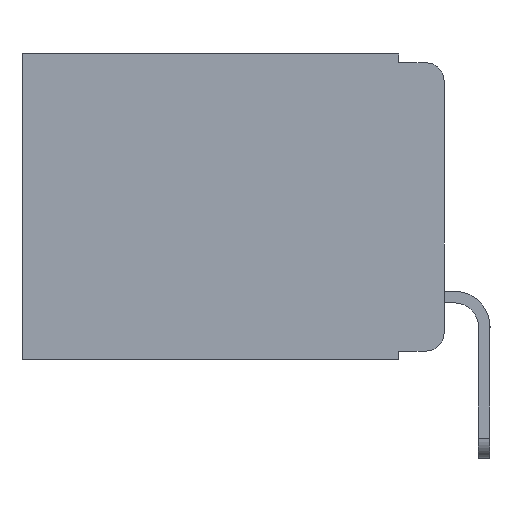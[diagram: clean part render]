
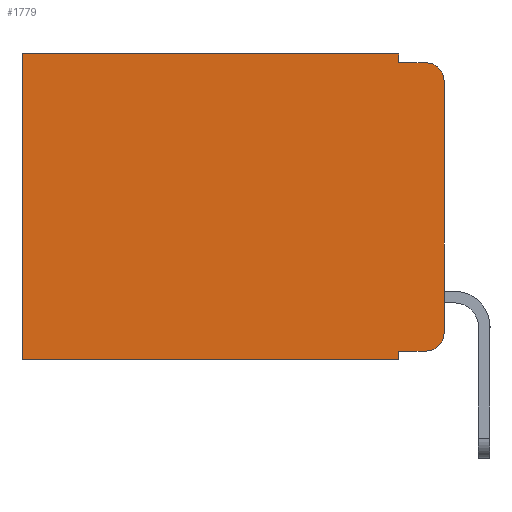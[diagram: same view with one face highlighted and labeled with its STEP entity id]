
A CAD part, left-side view. The second image highlights one B-rep face of the part: STEP entity #1779.
In plain terms, the highlighted planar face has unit normal (-1, 0, 0).
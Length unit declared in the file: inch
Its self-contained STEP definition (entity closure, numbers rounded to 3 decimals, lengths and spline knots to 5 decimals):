
#80 = CARTESIAN_POINT ( 'NONE',  ( 0.298, 0.473, 0. ) ) ;
#283 = FACE_OUTER_BOUND ( 'NONE', #10709, .T. ) ;
#819 = VERTEX_POINT ( 'NONE', #19769 ) ;
#1206 = LINE ( 'NONE', #15342, #15111 ) ;
#1315 = LINE ( 'NONE', #9828, #20934 ) ;
#1429 = CARTESIAN_POINT ( 'NONE',  ( 0.298, 0.02, -0.313 ) ) ;
#1667 = EDGE_CURVE ( 'NONE', #11596, #10722, #20579, .T. ) ;
#1669 = DIRECTION ( 'NONE',  ( -1., 0., 0. ) ) ;
#1767 = PLANE ( 'NONE',  #5149 ) ;
#1779 = ADVANCED_FACE ( 'NONE', ( #283 ), #1767, .F. ) ;
#2220 = ORIENTED_EDGE ( 'NONE', *, *, #22046, .F. ) ;
#2568 = CARTESIAN_POINT ( 'NONE',  ( 0.298, 0.051, 0. ) ) ;
#2847 = EDGE_CURVE ( 'NONE', #20224, #12367, #1315, .T. ) ;
#2848 = AXIS2_PLACEMENT_3D ( 'NONE', #6770, #5279, #20750 ) ;
#2864 = EDGE_CURVE ( 'NONE', #11699, #10668, #1206, .T. ) ;
#3841 = ORIENTED_EDGE ( 'NONE', *, *, #11175, .F. ) ;
#4038 = CARTESIAN_POINT ( 'NONE',  ( 0.298, 0.051, -0.01 ) ) ;
#4405 = VERTEX_POINT ( 'NONE', #10879 ) ;
#4861 = VECTOR ( 'NONE', #13452, 39.37008 ) ;
#5149 = AXIS2_PLACEMENT_3D ( 'NONE', #21024, #5321, #15904 ) ;
#5279 = DIRECTION ( 'NONE',  ( -1., 0., 0. ) ) ;
#5291 = VECTOR ( 'NONE', #14954, 39.37008 ) ;
#5321 = DIRECTION ( 'NONE',  ( 1., 0., 0. ) ) ;
#5646 = LINE ( 'NONE', #5753, #18004 ) ;
#5753 = CARTESIAN_POINT ( 'NONE',  ( 0.298, 0., 0. ) ) ;
#6373 = DIRECTION ( 'NONE',  ( 0., 0., -1. ) ) ;
#6407 = CARTESIAN_POINT ( 'NONE',  ( 0.298, 0.051, -0.333 ) ) ;
#6638 = CARTESIAN_POINT ( 'NONE',  ( 0.298, 0.473, 0. ) ) ;
#6770 = CARTESIAN_POINT ( 'NONE',  ( 0.298, 0.02, -0.03 ) ) ;
#6816 = EDGE_CURVE ( 'NONE', #11699, #11596, #7379, .T. ) ;
#6847 = CARTESIAN_POINT ( 'NONE',  ( 0.298, 0.473, -0.343 ) ) ;
#7379 = LINE ( 'NONE', #2568, #19168 ) ;
#7659 = ORIENTED_EDGE ( 'NONE', *, *, #6816, .F. ) ;
#7720 = ORIENTED_EDGE ( 'NONE', *, *, #21353, .T. ) ;
#8522 = VERTEX_POINT ( 'NONE', #16983 ) ;
#9321 = AXIS2_PLACEMENT_3D ( 'NONE', #1429, #1669, #17388 ) ;
#9828 = CARTESIAN_POINT ( 'NONE',  ( 0.298, 0.051, 0. ) ) ;
#10330 = ORIENTED_EDGE ( 'NONE', *, *, #11550, .T. ) ;
#10668 = VERTEX_POINT ( 'NONE', #22439 ) ;
#10709 = EDGE_LOOP ( 'NONE', ( #3841, #10330, #2220, #15737, #19781, #20776, #22475, #7659, #15639, #7720 ) ) ;
#10722 = VERTEX_POINT ( 'NONE', #6847 ) ;
#10879 = CARTESIAN_POINT ( 'NONE',  ( 0.298, 0., -0.03 ) ) ;
#11175 = EDGE_CURVE ( 'NONE', #4405, #8522, #5646, .T. ) ;
#11550 = EDGE_CURVE ( 'NONE', #4405, #819, #12733, .T. ) ;
#11596 = VERTEX_POINT ( 'NONE', #16418 ) ;
#11699 = VERTEX_POINT ( 'NONE', #6407 ) ;
#12367 = VERTEX_POINT ( 'NONE', #17274 ) ;
#12733 = CIRCLE ( 'NONE', #2848, 0.02 ) ;
#13181 = CARTESIAN_POINT ( 'NONE',  ( 0.298, 0.051, 0. ) ) ;
#13217 = VECTOR ( 'NONE', #16701, 39.37008 ) ;
#13341 = LINE ( 'NONE', #20218, #4861 ) ;
#13452 = DIRECTION ( 'NONE',  ( 0., 1., 0. ) ) ;
#14954 = DIRECTION ( 'NONE',  ( 0., -1., 0. ) ) ;
#15111 = VECTOR ( 'NONE', #20583, 39.37008 ) ;
#15220 = VERTEX_POINT ( 'NONE', #80 ) ;
#15337 = CARTESIAN_POINT ( 'NONE',  ( 0.298, 0., -0.343 ) ) ;
#15342 = CARTESIAN_POINT ( 'NONE',  ( 0.298, 0.051, -0.333 ) ) ;
#15639 = ORIENTED_EDGE ( 'NONE', *, *, #2864, .T. ) ;
#15737 = ORIENTED_EDGE ( 'NONE', *, *, #2847, .F. ) ;
#15904 = DIRECTION ( 'NONE',  ( 0., 0., -1. ) ) ;
#16311 = CIRCLE ( 'NONE', #9321, 0.02 ) ;
#16418 = CARTESIAN_POINT ( 'NONE',  ( 0.298, 0.051, -0.343 ) ) ;
#16553 = EDGE_CURVE ( 'NONE', #15220, #10722, #22335, .T. ) ;
#16701 = DIRECTION ( 'NONE',  ( 0., 1., 0. ) ) ;
#16983 = CARTESIAN_POINT ( 'NONE',  ( 0.298, 0., -0.313 ) ) ;
#17274 = CARTESIAN_POINT ( 'NONE',  ( 0.298, 0.051, -0.01 ) ) ;
#17388 = DIRECTION ( 'NONE',  ( 0., 0., -1. ) ) ;
#18004 = VECTOR ( 'NONE', #21232, 39.37008 ) ;
#18039 = LINE ( 'NONE', #4038, #5291 ) ;
#18078 = EDGE_CURVE ( 'NONE', #20224, #15220, #13341, .T. ) ;
#19168 = VECTOR ( 'NONE', #19551, 39.37008 ) ;
#19551 = DIRECTION ( 'NONE',  ( 0., 0., -1. ) ) ;
#19769 = CARTESIAN_POINT ( 'NONE',  ( 0.298, 0.02, -0.01 ) ) ;
#19781 = ORIENTED_EDGE ( 'NONE', *, *, #18078, .T. ) ;
#20218 = CARTESIAN_POINT ( 'NONE',  ( 0.298, 0., 0. ) ) ;
#20224 = VERTEX_POINT ( 'NONE', #13181 ) ;
#20579 = LINE ( 'NONE', #15337, #13217 ) ;
#20583 = DIRECTION ( 'NONE',  ( 0., -1., 0. ) ) ;
#20624 = DIRECTION ( 'NONE',  ( 0., 0., -1. ) ) ;
#20750 = DIRECTION ( 'NONE',  ( 0., 0., -1. ) ) ;
#20776 = ORIENTED_EDGE ( 'NONE', *, *, #16553, .T. ) ;
#20934 = VECTOR ( 'NONE', #6373, 39.37008 ) ;
#21024 = CARTESIAN_POINT ( 'NONE',  ( 0.298, 0., 0. ) ) ;
#21232 = DIRECTION ( 'NONE',  ( 0., 0., -1. ) ) ;
#21353 = EDGE_CURVE ( 'NONE', #10668, #8522, #16311, .T. ) ;
#22046 = EDGE_CURVE ( 'NONE', #12367, #819, #18039, .T. ) ;
#22335 = LINE ( 'NONE', #6638, #22375 ) ;
#22375 = VECTOR ( 'NONE', #20624, 39.37008 ) ;
#22439 = CARTESIAN_POINT ( 'NONE',  ( 0.298, 0.02, -0.333 ) ) ;
#22475 = ORIENTED_EDGE ( 'NONE', *, *, #1667, .F. ) ;
